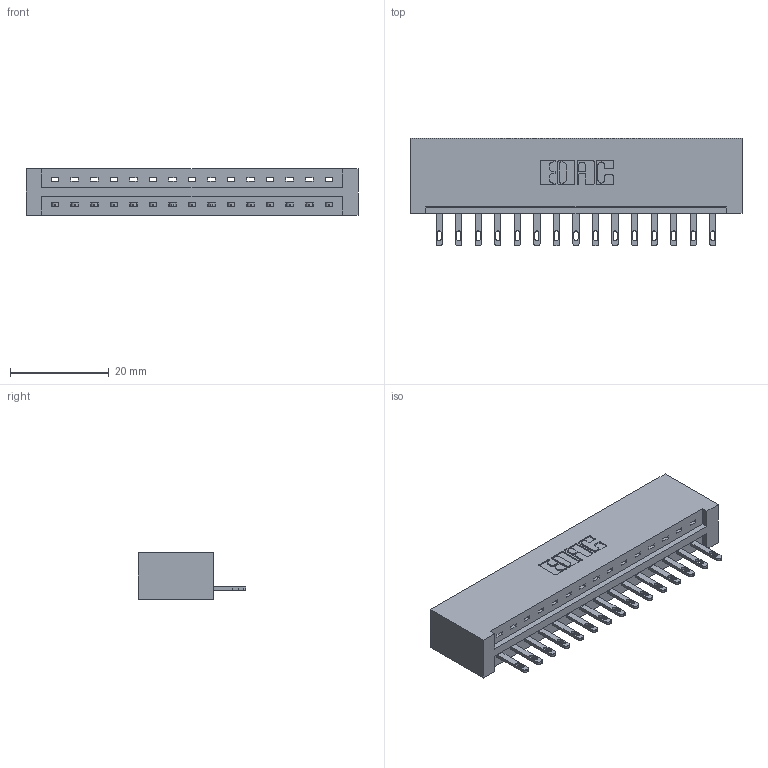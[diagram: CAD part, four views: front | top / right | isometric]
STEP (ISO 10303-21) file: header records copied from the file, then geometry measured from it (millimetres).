
FILE_DESCRIPTION (( 'STEP AP203' ), '1' );
FILE_NAME ('337-015-500-101.STEP', '2019-09-28T16:10:00', ( '' ), ( '' ), 'SwSTEP 2.0', 'SolidWorks 2016', '' );
FILE_SCHEMA (( 'CONFIG_CONTROL_DESIGN' ));
Length unit declared in the file: inch
Products named in the file (3): 345-292-001_345-293-100; 337-015-500-101; 337 Part_No Mounting Lugs
Assembly tree (16 placements, depth 2):
  337-015-500-101
    337 Part_No Mounting Lugs
    345-292-001_345-293-100  x15
Bounding box: 67.31 x 21.85 x 9.4 mm (x, y, z)
Volume: 7405.9 mm3; surface area: 7519.5 mm2
Topology: 16 solids, 16 shells, 976 faces, 2987 edges, 1990 vertices
Faces by surface type: plane 666, cylinder 310
Entity records: 14295 total; most frequent: CARTESIAN_POINT 2495, ORIENTED_EDGE 2446, DIRECTION 2149, EDGE_CURVE 1223, LINE 1099, VECTOR 1099, VERTEX_POINT 814, AXIS2_PLACEMENT_3D 525
